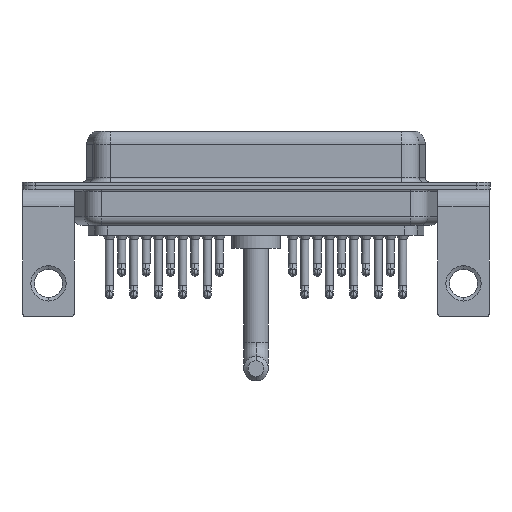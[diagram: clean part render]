
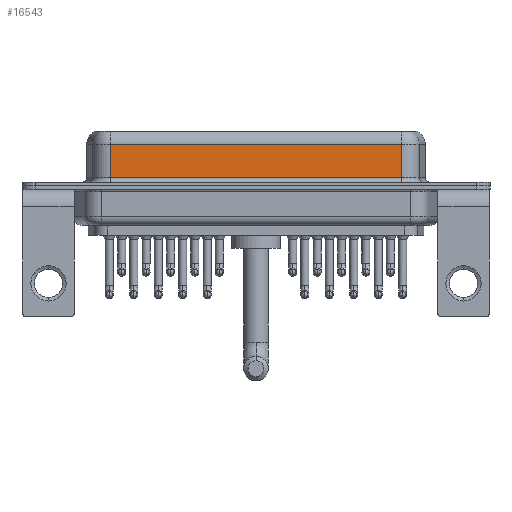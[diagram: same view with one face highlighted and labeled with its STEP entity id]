
A CAD part, front view. The second image highlights one B-rep face of the part: STEP entity #16543.
In plain terms, the highlighted planar face has unit normal (0, -1, 0).
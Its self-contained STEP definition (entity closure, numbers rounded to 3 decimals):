
#19 = CARTESIAN_POINT ( 'NONE',  ( 40.037, -3.95, 4.65 ) ) ;
#145 = VECTOR ( 'NONE', #4777, 1000. ) ;
#280 = VERTEX_POINT ( 'NONE', #22726 ) ;
#799 = ORIENTED_EDGE ( 'NONE', *, *, #18882, .T. ) ;
#1487 = CARTESIAN_POINT ( 'NONE',  ( 40.037, -3.95, 0.9 ) ) ;
#4777 = DIRECTION ( 'NONE',  ( 0., 0., -1. ) ) ;
#4819 = LINE ( 'NONE', #1487, #6173 ) ;
#5128 = CARTESIAN_POINT ( 'NONE',  ( 7.013, -3.95, 6.4 ) ) ;
#6124 = FACE_OUTER_BOUND ( 'NONE', #12851, .T. ) ;
#6173 = VECTOR ( 'NONE', #19749, 1000. ) ;
#6367 = LINE ( 'NONE', #11916, #10410 ) ;
#7774 = ORIENTED_EDGE ( 'NONE', *, *, #16708, .T. ) ;
#8371 = DIRECTION ( 'NONE',  ( -1., 0., 0. ) ) ;
#9181 = AXIS2_PLACEMENT_3D ( 'NONE', #18690, #11567, #15335 ) ;
#10410 = VECTOR ( 'NONE', #8371, 1000. ) ;
#10854 = ORIENTED_EDGE ( 'NONE', *, *, #12744, .T. ) ;
#11567 = DIRECTION ( 'NONE',  ( 0., 1., 0. ) ) ;
#11781 = ORIENTED_EDGE ( 'NONE', *, *, #13235, .F. ) ;
#11916 = CARTESIAN_POINT ( 'NONE',  ( 40.037, -3.95, 4.65 ) ) ;
#12304 = VERTEX_POINT ( 'NONE', #13943 ) ;
#12679 = CARTESIAN_POINT ( 'NONE',  ( 7.013, -3.95, 4.65 ) ) ;
#12744 = EDGE_CURVE ( 'NONE', #15352, #22036, #6367, .T. ) ;
#12851 = EDGE_LOOP ( 'NONE', ( #11781, #10854, #799, #7774 ) ) ;
#13235 = EDGE_CURVE ( 'NONE', #15352, #280, #13764, .T. ) ;
#13764 = LINE ( 'NONE', #19022, #14560 ) ;
#13943 = CARTESIAN_POINT ( 'NONE',  ( 7.013, -3.95, 0.9 ) ) ;
#14094 = LINE ( 'NONE', #5128, #145 ) ;
#14560 = VECTOR ( 'NONE', #21029, 1000. ) ;
#14992 = PLANE ( 'NONE',  #9181 ) ;
#15335 = DIRECTION ( 'NONE',  ( 0., 0., 1. ) ) ;
#15352 = VERTEX_POINT ( 'NONE', #19 ) ;
#16543 = ADVANCED_FACE ( 'NONE', ( #6124 ), #14992, .F. ) ;
#16708 = EDGE_CURVE ( 'NONE', #12304, #280, #4819, .T. ) ;
#18690 = CARTESIAN_POINT ( 'NONE',  ( 40.037, -3.95, 6.4 ) ) ;
#18882 = EDGE_CURVE ( 'NONE', #22036, #12304, #14094, .T. ) ;
#19022 = CARTESIAN_POINT ( 'NONE',  ( 40.037, -3.95, 6.4 ) ) ;
#19749 = DIRECTION ( 'NONE',  ( 1., 0., 0. ) ) ;
#21029 = DIRECTION ( 'NONE',  ( 0., 0., -1. ) ) ;
#22036 = VERTEX_POINT ( 'NONE', #12679 ) ;
#22726 = CARTESIAN_POINT ( 'NONE',  ( 40.037, -3.95, 0.9 ) ) ;
